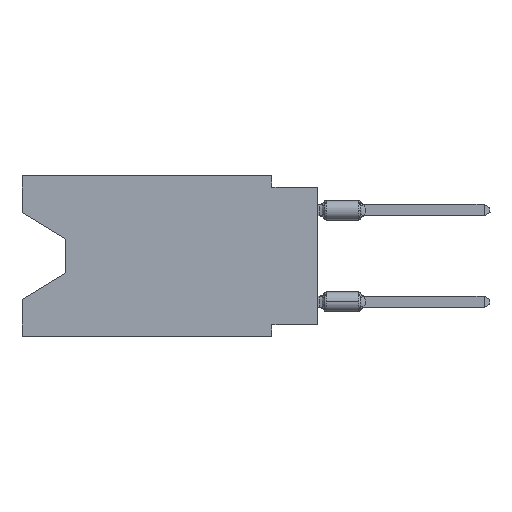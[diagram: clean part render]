
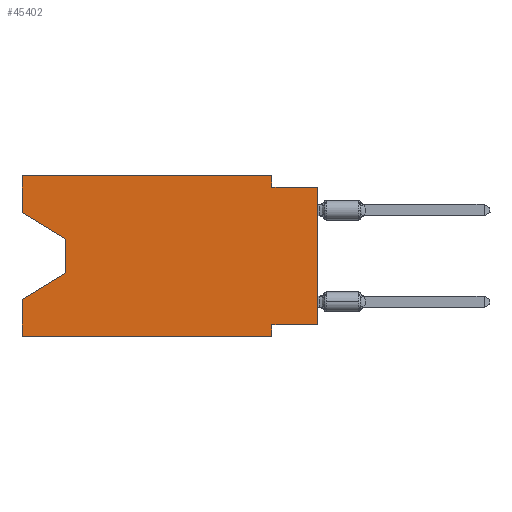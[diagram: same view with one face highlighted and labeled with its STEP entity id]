
A CAD part, left-side view. The second image highlights one B-rep face of the part: STEP entity #45402.
In plain terms, the highlighted planar face has unit normal (-1, 0, 0).
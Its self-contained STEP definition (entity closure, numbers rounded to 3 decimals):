
#374 = VECTOR ( 'NONE', #40356, 1000. ) ;
#1257 = CARTESIAN_POINT ( 'NONE',  ( 0., 16.383, -8.89 ) ) ;
#1328 = ORIENTED_EDGE ( 'NONE', *, *, #19830, .T. ) ;
#1568 = CARTESIAN_POINT ( 'NONE',  ( 0., 0., -0.635 ) ) ;
#1849 = DIRECTION ( 'NONE',  ( 0., -1., 0. ) ) ;
#2657 = VERTEX_POINT ( 'NONE', #38108 ) ;
#3846 = VERTEX_POINT ( 'NONE', #12545 ) ;
#5401 = VERTEX_POINT ( 'NONE', #1568 ) ;
#5512 = VECTOR ( 'NONE', #24597, 1000. ) ;
#6960 = EDGE_CURVE ( 'NONE', #21106, #8543, #26356, .T. ) ;
#7017 = CARTESIAN_POINT ( 'NONE',  ( 0., 2.54, -8.255 ) ) ;
#7066 = EDGE_CURVE ( 'NONE', #11236, #2657, #20853, .T. ) ;
#7105 = VECTOR ( 'NONE', #36324, 1000. ) ;
#7309 = CARTESIAN_POINT ( 'NONE',  ( 0., 16.383, 0. ) ) ;
#7835 = CARTESIAN_POINT ( 'NONE',  ( 0., 13.97, -5.385 ) ) ;
#8543 = VERTEX_POINT ( 'NONE', #33983 ) ;
#8879 = EDGE_CURVE ( 'NONE', #46942, #3846, #12607, .T. ) ;
#10703 = EDGE_CURVE ( 'NONE', #46871, #21106, #13556, .T. ) ;
#10791 = DIRECTION ( 'NONE',  ( 0., 0., 1. ) ) ;
#11127 = ORIENTED_EDGE ( 'NONE', *, *, #44857, .F. ) ;
#11140 = VERTEX_POINT ( 'NONE', #21896 ) ;
#11236 = VERTEX_POINT ( 'NONE', #26125 ) ;
#11843 = ORIENTED_EDGE ( 'NONE', *, *, #23645, .T. ) ;
#12545 = CARTESIAN_POINT ( 'NONE',  ( 0., 2.54, -8.89 ) ) ;
#12607 = LINE ( 'NONE', #20792, #23115 ) ;
#13241 = EDGE_LOOP ( 'NONE', ( #27220, #15670, #11843, #39122, #1328, #21908, #16396, #46469, #34420, #39026, #23216, #11127 ) ) ;
#13263 = VECTOR ( 'NONE', #28695, 1000. ) ;
#13556 = LINE ( 'NONE', #14278, #13263 ) ;
#13800 = VECTOR ( 'NONE', #39440, 1000. ) ;
#14278 = CARTESIAN_POINT ( 'NONE',  ( 0., 16.383, 0. ) ) ;
#14721 = PLANE ( 'NONE',  #32156 ) ;
#15126 = LINE ( 'NONE', #45170, #36773 ) ;
#15670 = ORIENTED_EDGE ( 'NONE', *, *, #20426, .T. ) ;
#16303 = VECTOR ( 'NONE', #10791, 1000. ) ;
#16396 = ORIENTED_EDGE ( 'NONE', *, *, #43974, .F. ) ;
#17108 = DIRECTION ( 'NONE',  ( 0., 0., -1. ) ) ;
#17704 = LINE ( 'NONE', #21445, #7105 ) ;
#17727 = CARTESIAN_POINT ( 'NONE',  ( 0., 16.383, -2.038 ) ) ;
#19830 = EDGE_CURVE ( 'NONE', #11236, #3846, #39709, .T. ) ;
#19871 = CARTESIAN_POINT ( 'NONE',  ( 0., 13.97, -5.385 ) ) ;
#20426 = EDGE_CURVE ( 'NONE', #35752, #28850, #17704, .T. ) ;
#20792 = CARTESIAN_POINT ( 'NONE',  ( 0., 2.54, -8.89 ) ) ;
#20853 = LINE ( 'NONE', #28313, #5512 ) ;
#21106 = VERTEX_POINT ( 'NONE', #35465 ) ;
#21445 = CARTESIAN_POINT ( 'NONE',  ( 0., 13.97, -3.505 ) ) ;
#21896 = CARTESIAN_POINT ( 'NONE',  ( 0., 0., -8.255 ) ) ;
#21908 = ORIENTED_EDGE ( 'NONE', *, *, #8879, .F. ) ;
#22430 = DIRECTION ( 'NONE',  ( 1., 0., 0. ) ) ;
#23115 = VECTOR ( 'NONE', #35914, 1000. ) ;
#23216 = ORIENTED_EDGE ( 'NONE', *, *, #10703, .F. ) ;
#23645 = EDGE_CURVE ( 'NONE', #28850, #2657, #35972, .T. ) ;
#24597 = DIRECTION ( 'NONE',  ( 0., 0., 1. ) ) ;
#25503 = CARTESIAN_POINT ( 'NONE',  ( 0., 16.383, 0. ) ) ;
#26125 = CARTESIAN_POINT ( 'NONE',  ( 0., 16.383, -8.89 ) ) ;
#26356 = LINE ( 'NONE', #34276, #31649 ) ;
#26861 = VECTOR ( 'NONE', #28314, 1000. ) ;
#27220 = ORIENTED_EDGE ( 'NONE', *, *, #45585, .T. ) ;
#27924 = VERTEX_POINT ( 'NONE', #17727 ) ;
#28313 = CARTESIAN_POINT ( 'NONE',  ( 0., 16.383, 0. ) ) ;
#28314 = DIRECTION ( 'NONE',  ( 0., -1., 0. ) ) ;
#28695 = DIRECTION ( 'NONE',  ( 0., -1., 0. ) ) ;
#28850 = VERTEX_POINT ( 'NONE', #7835 ) ;
#29027 = CARTESIAN_POINT ( 'NONE',  ( 0., 16.383, -2.038 ) ) ;
#29757 = DIRECTION ( 'NONE',  ( 0., -0.855, -0.519 ) ) ;
#30391 = LINE ( 'NONE', #37819, #16303 ) ;
#30708 = VECTOR ( 'NONE', #1849, 1000. ) ;
#31622 = LINE ( 'NONE', #35827, #30708 ) ;
#31649 = VECTOR ( 'NONE', #41459, 1000. ) ;
#32156 = AXIS2_PLACEMENT_3D ( 'NONE', #7309, #22430, #17108 ) ;
#32944 = EDGE_CURVE ( 'NONE', #11140, #5401, #30391, .T. ) ;
#33983 = CARTESIAN_POINT ( 'NONE',  ( 0., 2.54, -0.635 ) ) ;
#33986 = DIRECTION ( 'NONE',  ( 0., 1., 0. ) ) ;
#34276 = CARTESIAN_POINT ( 'NONE',  ( 0., 2.54, 0. ) ) ;
#34390 = EDGE_CURVE ( 'NONE', #8543, #5401, #31622, .T. ) ;
#34420 = ORIENTED_EDGE ( 'NONE', *, *, #34390, .F. ) ;
#35465 = CARTESIAN_POINT ( 'NONE',  ( 0., 2.54, 0. ) ) ;
#35752 = VERTEX_POINT ( 'NONE', #44016 ) ;
#35827 = CARTESIAN_POINT ( 'NONE',  ( 0., 0., -0.635 ) ) ;
#35914 = DIRECTION ( 'NONE',  ( 0., 0., -1. ) ) ;
#35972 = LINE ( 'NONE', #19871, #13800 ) ;
#36324 = DIRECTION ( 'NONE',  ( 0., 0., -1. ) ) ;
#36773 = VECTOR ( 'NONE', #33986, 1000. ) ;
#37819 = CARTESIAN_POINT ( 'NONE',  ( 0., 0., 0. ) ) ;
#38108 = CARTESIAN_POINT ( 'NONE',  ( 0., 16.383, -6.852 ) ) ;
#39026 = ORIENTED_EDGE ( 'NONE', *, *, #6960, .F. ) ;
#39122 = ORIENTED_EDGE ( 'NONE', *, *, #7066, .F. ) ;
#39440 = DIRECTION ( 'NONE',  ( 0., 0.855, -0.519 ) ) ;
#39709 = LINE ( 'NONE', #1257, #26861 ) ;
#39758 = CARTESIAN_POINT ( 'NONE',  ( 0., 16.383, 0. ) ) ;
#40356 = DIRECTION ( 'NONE',  ( 0., 0., 1. ) ) ;
#41459 = DIRECTION ( 'NONE',  ( 0., 0., -1. ) ) ;
#43974 = EDGE_CURVE ( 'NONE', #11140, #46942, #15126, .T. ) ;
#44016 = CARTESIAN_POINT ( 'NONE',  ( 0., 13.97, -3.505 ) ) ;
#44087 = LINE ( 'NONE', #25503, #374 ) ;
#44857 = EDGE_CURVE ( 'NONE', #27924, #46871, #44087, .T. ) ;
#44889 = LINE ( 'NONE', #29027, #45611 ) ;
#45170 = CARTESIAN_POINT ( 'NONE',  ( 0., 0., -8.255 ) ) ;
#45402 = ADVANCED_FACE ( 'NONE', ( #48766 ), #14721, .F. ) ;
#45585 = EDGE_CURVE ( 'NONE', #27924, #35752, #44889, .T. ) ;
#45611 = VECTOR ( 'NONE', #29757, 1000. ) ;
#46469 = ORIENTED_EDGE ( 'NONE', *, *, #32944, .T. ) ;
#46871 = VERTEX_POINT ( 'NONE', #39758 ) ;
#46942 = VERTEX_POINT ( 'NONE', #7017 ) ;
#48766 = FACE_OUTER_BOUND ( 'NONE', #13241, .T. ) ;
